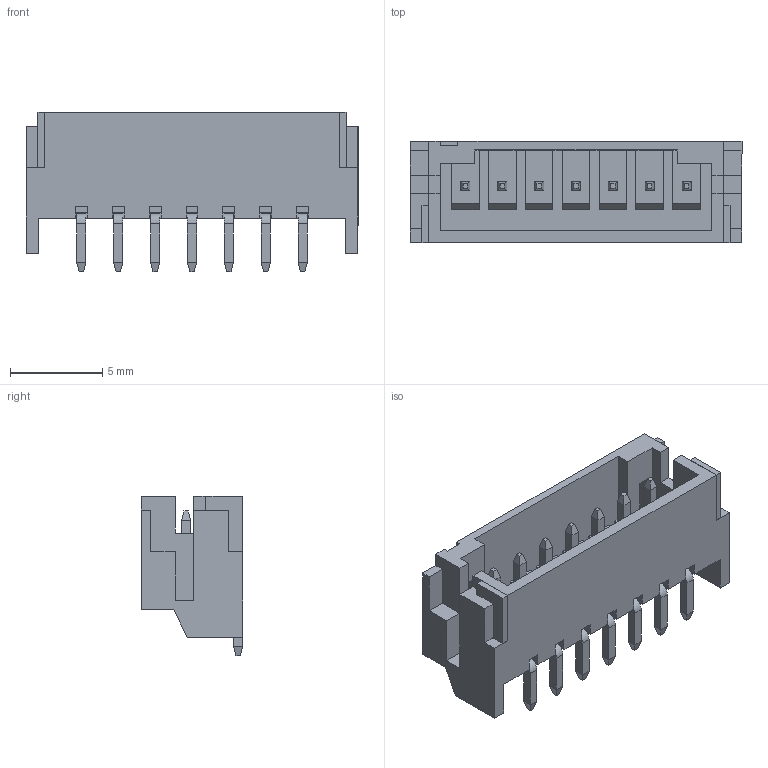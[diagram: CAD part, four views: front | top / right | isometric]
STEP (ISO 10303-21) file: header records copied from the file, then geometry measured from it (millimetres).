
FILE_DESCRIPTION (( 'STEP AP203' ), '1' );
FILE_NAME ('140-507-417-060.STEP', '2020-03-31T20:21:35', ( '' ), ( '' ), 'SwSTEP 2.0', 'SolidWorks 2016', '' );
FILE_SCHEMA (( 'CONFIG_CONTROL_DESIGN' ));
Length unit declared in the file: millimetre
Products named in the file (4): RA SMT Housing_507; RA SMT Contact; RA SMT Pad; 140-507-417-060
Assembly tree (10 placements, depth 2):
  140-507-417-060
    RA SMT Housing_507
    RA SMT Contact  x7
    RA SMT Pad  x2
Bounding box: 18 x 5.5 x 8.65 mm (x, y, z)
Volume: 258.2 mm3; surface area: 955.2 mm2
Topology: 10 solids, 10 shells, 402 faces, 988 edges, 602 vertices
Faces by surface type: plane 374, cylinder 28
Entity records: 7534 total; most frequent: CARTESIAN_POINT 1247, ORIENTED_EDGE 1232, DIRECTION 1082, EDGE_CURVE 616, VECTOR 608, LINE 608, VERTEX_POINT 402, AXIS2_PLACEMENT_3D 237
